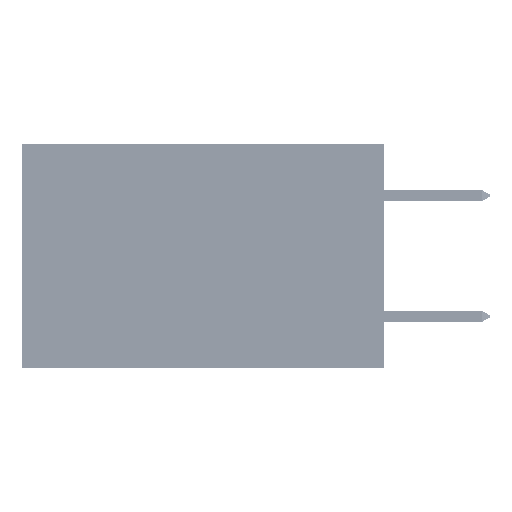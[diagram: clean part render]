
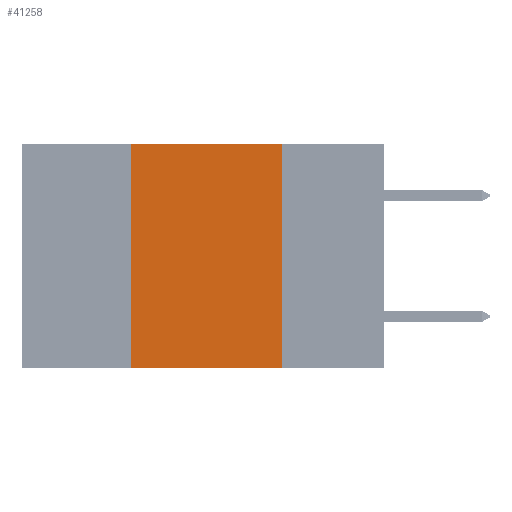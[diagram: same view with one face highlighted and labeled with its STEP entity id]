
A CAD part, left-side view. The second image highlights one B-rep face of the part: STEP entity #41258.
In plain terms, the highlighted planar face has unit normal (-1, 0, 0).
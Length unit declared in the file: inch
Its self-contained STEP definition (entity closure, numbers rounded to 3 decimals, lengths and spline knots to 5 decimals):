
#700 = DIRECTION ( 'NONE',  ( 0., -1., 0. ) ) ;
#5036 = CARTESIAN_POINT ( 'NONE',  ( 0., 0.17, 0. ) ) ;
#5956 = LINE ( 'NONE', #7528, #43992 ) ;
#7528 = CARTESIAN_POINT ( 'NONE',  ( 0., 0.42, 0. ) ) ;
#9467 = VECTOR ( 'NONE', #19236, 39.37008 ) ;
#9597 = CARTESIAN_POINT ( 'NONE',  ( 0., 0.42, 0. ) ) ;
#14441 = DIRECTION ( 'NONE',  ( 1., 0., 0. ) ) ;
#14914 = PLANE ( 'NONE',  #29648 ) ;
#16765 = DIRECTION ( 'NONE',  ( 0., 0., -1. ) ) ;
#17736 = EDGE_CURVE ( 'NONE', #31569, #40177, #31797, .T. ) ;
#17740 = ORIENTED_EDGE ( 'NONE', *, *, #17736, .F. ) ;
#18023 = CARTESIAN_POINT ( 'NONE',  ( 0., 0.6, 0. ) ) ;
#18124 = CARTESIAN_POINT ( 'NONE',  ( 0., 0.6, -0.37 ) ) ;
#18775 = ORIENTED_EDGE ( 'NONE', *, *, #31657, .F. ) ;
#19236 = DIRECTION ( 'NONE',  ( 0., -1., 0. ) ) ;
#22236 = EDGE_CURVE ( 'NONE', #42265, #28450, #42330, .T. ) ;
#23004 = CARTESIAN_POINT ( 'NONE',  ( 0., 0.17, -0.37 ) ) ;
#25301 = ORIENTED_EDGE ( 'NONE', *, *, #22236, .T. ) ;
#27673 = CARTESIAN_POINT ( 'NONE',  ( 0., 0.17, 0. ) ) ;
#28450 = VERTEX_POINT ( 'NONE', #23004 ) ;
#28862 = VECTOR ( 'NONE', #16765, 39.37008 ) ;
#29095 = DIRECTION ( 'NONE',  ( 0., 0., 1. ) ) ;
#29648 = AXIS2_PLACEMENT_3D ( 'NONE', #18023, #14441, #40089 ) ;
#30505 = LINE ( 'NONE', #27673, #28862 ) ;
#31191 = ORIENTED_EDGE ( 'NONE', *, *, #37963, .F. ) ;
#31569 = VERTEX_POINT ( 'NONE', #9597 ) ;
#31657 = EDGE_CURVE ( 'NONE', #40177, #28450, #30505, .T. ) ;
#31797 = LINE ( 'NONE', #33922, #9467 ) ;
#33402 = VECTOR ( 'NONE', #700, 39.37008 ) ;
#33922 = CARTESIAN_POINT ( 'NONE',  ( 0., 0.6, 0. ) ) ;
#35780 = FACE_OUTER_BOUND ( 'NONE', #36933, .T. ) ;
#36933 = EDGE_LOOP ( 'NONE', ( #18775, #17740, #31191, #25301 ) ) ;
#37963 = EDGE_CURVE ( 'NONE', #42265, #31569, #5956, .T. ) ;
#40089 = DIRECTION ( 'NONE',  ( 0., 0., -1. ) ) ;
#40177 = VERTEX_POINT ( 'NONE', #5036 ) ;
#41258 = ADVANCED_FACE ( 'NONE', ( #35780 ), #14914, .F. ) ;
#42265 = VERTEX_POINT ( 'NONE', #44327 ) ;
#42330 = LINE ( 'NONE', #18124, #33402 ) ;
#43992 = VECTOR ( 'NONE', #29095, 39.37008 ) ;
#44327 = CARTESIAN_POINT ( 'NONE',  ( 0., 0.42, -0.37 ) ) ;
